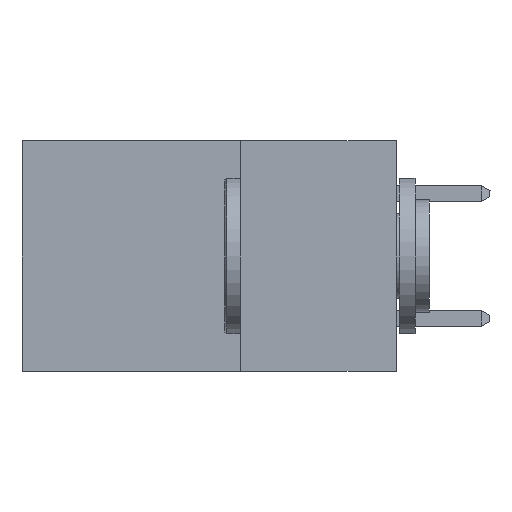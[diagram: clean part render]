
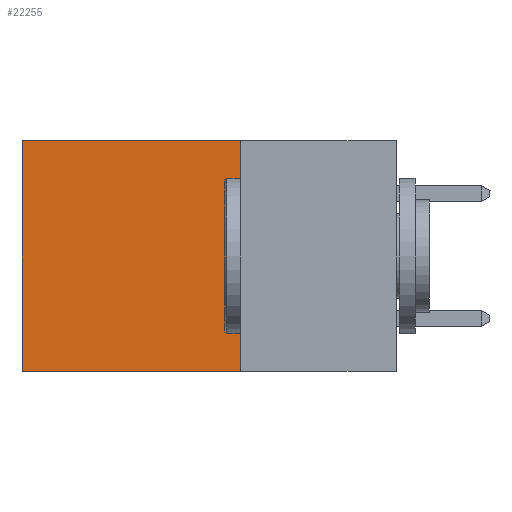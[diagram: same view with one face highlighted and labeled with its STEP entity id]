
A CAD part, left-side view. The second image highlights one B-rep face of the part: STEP entity #22255.
In plain terms, the highlighted planar face has unit normal (-1, 0, 0).
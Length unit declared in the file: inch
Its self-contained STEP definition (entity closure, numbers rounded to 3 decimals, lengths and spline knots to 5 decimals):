
#1588 = CARTESIAN_POINT ( 'NONE',  ( 0.2615, 0.25, -0.37 ) ) ;
#1629 = EDGE_CURVE ( 'NONE', #11713, #19342, #27320, .T. ) ;
#1889 = CARTESIAN_POINT ( 'NONE',  ( 0.2615, 0.6, -0.37 ) ) ;
#2094 = CARTESIAN_POINT ( 'NONE',  ( 0.2615, 0.25, 0. ) ) ;
#2845 = VERTEX_POINT ( 'NONE', #1889 ) ;
#4530 = VECTOR ( 'NONE', #5098, 39.37008 ) ;
#4918 = VECTOR ( 'NONE', #8648, 39.37008 ) ;
#5098 = DIRECTION ( 'NONE',  ( 0., 0., -1. ) ) ;
#5623 = EDGE_CURVE ( 'NONE', #19342, #2845, #22775, .T. ) ;
#5932 = ORIENTED_EDGE ( 'NONE', *, *, #10285, .T. ) ;
#8330 = LINE ( 'NONE', #12358, #24861 ) ;
#8648 = DIRECTION ( 'NONE',  ( 0., 1., 0. ) ) ;
#10285 = EDGE_CURVE ( 'NONE', #19844, #2845, #22641, .T. ) ;
#10518 = PLANE ( 'NONE',  #26603 ) ;
#10950 = ORIENTED_EDGE ( 'NONE', *, *, #5623, .F. ) ;
#11713 = VERTEX_POINT ( 'NONE', #2094 ) ;
#12238 = EDGE_CURVE ( 'NONE', #11713, #19844, #8330, .T. ) ;
#12358 = CARTESIAN_POINT ( 'NONE',  ( 0.2615, 0.25, 0. ) ) ;
#12713 = DIRECTION ( 'NONE',  ( 1., 0., 0. ) ) ;
#13130 = ORIENTED_EDGE ( 'NONE', *, *, #1629, .F. ) ;
#13454 = ORIENTED_EDGE ( 'NONE', *, *, #12238, .T. ) ;
#14518 = DIRECTION ( 'NONE',  ( 0., 1., 0. ) ) ;
#15168 = CARTESIAN_POINT ( 'NONE',  ( 0.2615, 0.25, -0.37 ) ) ;
#16888 = VECTOR ( 'NONE', #19351, 39.37008 ) ;
#17159 = CARTESIAN_POINT ( 'NONE',  ( 0.2615, 0.6, -0.37 ) ) ;
#18286 = CARTESIAN_POINT ( 'NONE',  ( 0.2615, 0.25, -0.37 ) ) ;
#19342 = VERTEX_POINT ( 'NONE', #18286 ) ;
#19351 = DIRECTION ( 'NONE',  ( 0., 0., -1. ) ) ;
#19844 = VERTEX_POINT ( 'NONE', #26675 ) ;
#22255 = ADVANCED_FACE ( 'NONE', ( #25190 ), #10518, .F. ) ;
#22472 = EDGE_LOOP ( 'NONE', ( #5932, #10950, #13130, #13454 ) ) ;
#22641 = LINE ( 'NONE', #17159, #16888 ) ;
#22775 = LINE ( 'NONE', #15168, #4918 ) ;
#23477 = CARTESIAN_POINT ( 'NONE',  ( 0.2615, 0.25, -0.37 ) ) ;
#24861 = VECTOR ( 'NONE', #14518, 39.37008 ) ;
#25190 = FACE_OUTER_BOUND ( 'NONE', #22472, .T. ) ;
#26603 = AXIS2_PLACEMENT_3D ( 'NONE', #23477, #12713, #27672 ) ;
#26675 = CARTESIAN_POINT ( 'NONE',  ( 0.2615, 0.6, 0. ) ) ;
#27320 = LINE ( 'NONE', #1588, #4530 ) ;
#27672 = DIRECTION ( 'NONE',  ( 0., 0., -1. ) ) ;
